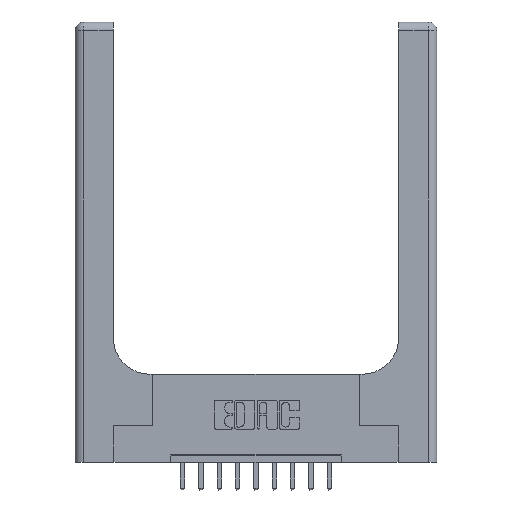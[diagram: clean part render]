
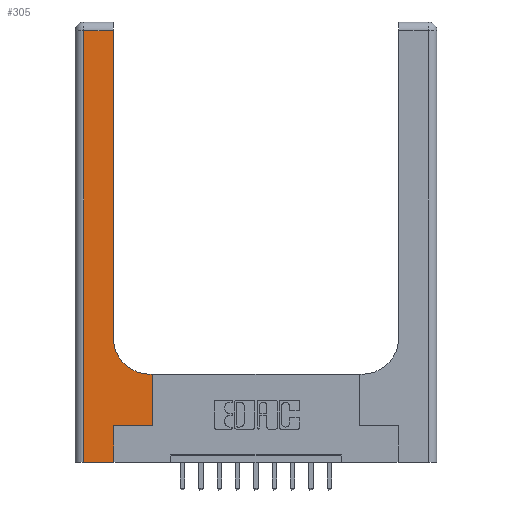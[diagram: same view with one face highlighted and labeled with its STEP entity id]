
A CAD part, top view. The second image highlights one B-rep face of the part: STEP entity #305.
In plain terms, the highlighted planar face has unit normal (0, 0, 1).
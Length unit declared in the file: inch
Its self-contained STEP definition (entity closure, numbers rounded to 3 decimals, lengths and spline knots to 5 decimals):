
#110 = VERTEX_POINT ( 'NONE', #14172 ) ;
#305 = ADVANCED_FACE ( 'NONE', ( #7771 ), #12170, .F. ) ;
#460 = ORIENTED_EDGE ( 'NONE', *, *, #3972, .T. ) ;
#652 = EDGE_CURVE ( 'NONE', #14021, #6736, #8520, .T. ) ;
#679 = DIRECTION ( 'NONE',  ( -1., 0., 0. ) ) ;
#957 = ORIENTED_EDGE ( 'NONE', *, *, #652, .T. ) ;
#1201 = CARTESIAN_POINT ( 'NONE',  ( 0.26, 3., 0.37 ) ) ;
#1252 = DIRECTION ( 'NONE',  ( 1., 0., 0. ) ) ;
#1603 = DIRECTION ( 'NONE',  ( -1., 0., 0. ) ) ;
#2152 = ORIENTED_EDGE ( 'NONE', *, *, #7066, .T. ) ;
#2210 = CARTESIAN_POINT ( 'NONE',  ( 0.51, 0.6, 0.37 ) ) ;
#2334 = CARTESIAN_POINT ( 'NONE',  ( 0.528, 0.25, 0.37 ) ) ;
#2506 = CARTESIAN_POINT ( 'NONE',  ( 0.265, 0., 0.37 ) ) ;
#2523 = EDGE_LOOP ( 'NONE', ( #2152, #8897, #957, #3420, #5593, #8750, #10455, #9647, #460 ) ) ;
#2567 = CARTESIAN_POINT ( 'NONE',  ( 0.528, 0.6, 0.37 ) ) ;
#2571 = VERTEX_POINT ( 'NONE', #2567 ) ;
#2968 = VECTOR ( 'NONE', #10245, 39.37008 ) ;
#3190 = VECTOR ( 'NONE', #11186, 39.37008 ) ;
#3257 = VERTEX_POINT ( 'NONE', #7320 ) ;
#3282 = CARTESIAN_POINT ( 'NONE',  ( 0.26, 2.94, 0.37 ) ) ;
#3420 = ORIENTED_EDGE ( 'NONE', *, *, #7954, .T. ) ;
#3447 = DIRECTION ( 'NONE',  ( 0., 0., -1. ) ) ;
#3748 = CIRCLE ( 'NONE', #13726, 0.25 ) ;
#3972 = EDGE_CURVE ( 'NONE', #9896, #3257, #3748, .T. ) ;
#4216 = LINE ( 'NONE', #2334, #5355 ) ;
#4661 = VECTOR ( 'NONE', #7110, 39.37008 ) ;
#4784 = DIRECTION ( 'NONE',  ( 1., 0., 0. ) ) ;
#4867 = EDGE_CURVE ( 'NONE', #5217, #110, #7842, .T. ) ;
#5217 = VERTEX_POINT ( 'NONE', #2506 ) ;
#5355 = VECTOR ( 'NONE', #10692, 39.37008 ) ;
#5423 = EDGE_CURVE ( 'NONE', #13298, #14021, #9980, .T. ) ;
#5482 = CARTESIAN_POINT ( 'NONE',  ( 0.528, 0.25, 0.37 ) ) ;
#5593 = ORIENTED_EDGE ( 'NONE', *, *, #4867, .T. ) ;
#5847 = VECTOR ( 'NONE', #14822, 39.37008 ) ;
#6736 = VERTEX_POINT ( 'NONE', #9169 ) ;
#7066 = EDGE_CURVE ( 'NONE', #3257, #13298, #11574, .T. ) ;
#7110 = DIRECTION ( 'NONE',  ( 0., 1., 0. ) ) ;
#7320 = CARTESIAN_POINT ( 'NONE',  ( 0.26, 0.85, 0.37 ) ) ;
#7741 = CARTESIAN_POINT ( 'NONE',  ( 0., 2.94, 0.37 ) ) ;
#7771 = FACE_OUTER_BOUND ( 'NONE', #2523, .T. ) ;
#7842 = LINE ( 'NONE', #12433, #3190 ) ;
#7918 = VECTOR ( 'NONE', #1252, 39.37008 ) ;
#7925 = VERTEX_POINT ( 'NONE', #5482 ) ;
#7954 = EDGE_CURVE ( 'NONE', #6736, #5217, #8563, .T. ) ;
#7965 = CARTESIAN_POINT ( 'NONE',  ( 0.26, 0.6, 0.37 ) ) ;
#8520 = LINE ( 'NONE', #11691, #9291 ) ;
#8563 = LINE ( 'NONE', #11372, #2968 ) ;
#8635 = DIRECTION ( 'NONE',  ( 0., 0., -1. ) ) ;
#8647 = LINE ( 'NONE', #7965, #11094 ) ;
#8750 = ORIENTED_EDGE ( 'NONE', *, *, #13163, .T. ) ;
#8897 = ORIENTED_EDGE ( 'NONE', *, *, #5423, .T. ) ;
#9122 = CARTESIAN_POINT ( 'NONE',  ( 0.06, 2.94, 0.37 ) ) ;
#9169 = CARTESIAN_POINT ( 'NONE',  ( 0.06, 0., 0.37 ) ) ;
#9181 = EDGE_CURVE ( 'NONE', #7925, #2571, #4216, .T. ) ;
#9291 = VECTOR ( 'NONE', #14099, 39.37008 ) ;
#9647 = ORIENTED_EDGE ( 'NONE', *, *, #13669, .T. ) ;
#9896 = VERTEX_POINT ( 'NONE', #2210 ) ;
#9980 = LINE ( 'NONE', #7741, #5847 ) ;
#10245 = DIRECTION ( 'NONE',  ( 1., 0., 0. ) ) ;
#10455 = ORIENTED_EDGE ( 'NONE', *, *, #9181, .T. ) ;
#10679 = AXIS2_PLACEMENT_3D ( 'NONE', #11158, #8635, #1603 ) ;
#10692 = DIRECTION ( 'NONE',  ( 0., 1., 0. ) ) ;
#11094 = VECTOR ( 'NONE', #679, 39.37008 ) ;
#11158 = CARTESIAN_POINT ( 'NONE',  ( 0., 3., 0.37 ) ) ;
#11186 = DIRECTION ( 'NONE',  ( 0., 1., 0. ) ) ;
#11372 = CARTESIAN_POINT ( 'NONE',  ( 0., 0., 0.37 ) ) ;
#11574 = LINE ( 'NONE', #1201, #4661 ) ;
#11691 = CARTESIAN_POINT ( 'NONE',  ( 0.06, 3., 0.37 ) ) ;
#12170 = PLANE ( 'NONE',  #10679 ) ;
#12433 = CARTESIAN_POINT ( 'NONE',  ( 0.265, 0., 0.37 ) ) ;
#13109 = CARTESIAN_POINT ( 'NONE',  ( 0.51, 0.85, 0.37 ) ) ;
#13163 = EDGE_CURVE ( 'NONE', #110, #7925, #14222, .T. ) ;
#13298 = VERTEX_POINT ( 'NONE', #3282 ) ;
#13669 = EDGE_CURVE ( 'NONE', #2571, #9896, #8647, .T. ) ;
#13726 = AXIS2_PLACEMENT_3D ( 'NONE', #13109, #3447, #4784 ) ;
#14021 = VERTEX_POINT ( 'NONE', #9122 ) ;
#14099 = DIRECTION ( 'NONE',  ( 0., -1., 0. ) ) ;
#14172 = CARTESIAN_POINT ( 'NONE',  ( 0.265, 0.25, 0.37 ) ) ;
#14222 = LINE ( 'NONE', #14274, #7918 ) ;
#14274 = CARTESIAN_POINT ( 'NONE',  ( 0.265, 0.25, 0.37 ) ) ;
#14822 = DIRECTION ( 'NONE',  ( -1., 0., 0. ) ) ;
